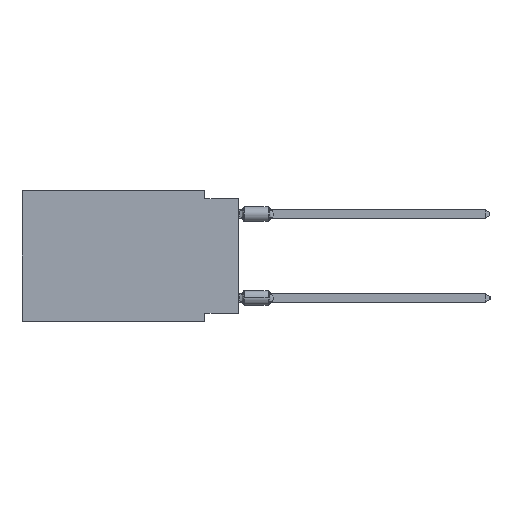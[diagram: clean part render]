
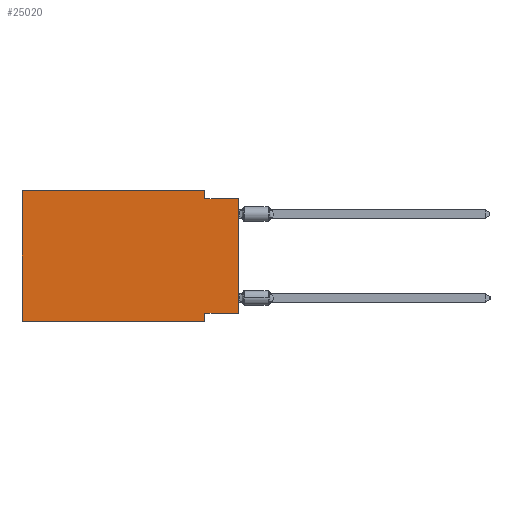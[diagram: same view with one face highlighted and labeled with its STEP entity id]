
A CAD part, left-side view. The second image highlights one B-rep face of the part: STEP entity #25020.
In plain terms, the highlighted planar face has unit normal (-1, 0, 0).
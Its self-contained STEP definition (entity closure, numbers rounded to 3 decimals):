
#101 = EDGE_CURVE ( 'NONE', #22344, #44225, #12559, .T. ) ;
#340 = AXIS2_PLACEMENT_3D ( 'NONE', #10035, #46020, #37807 ) ;
#883 = DIRECTION ( 'NONE',  ( 0., 0., 1. ) ) ;
#992 = EDGE_CURVE ( 'NONE', #17172, #22344, #31655, .T. ) ;
#3326 = CARTESIAN_POINT ( 'NONE',  ( 0., 2.54, -0.635 ) ) ;
#3798 = VERTEX_POINT ( 'NONE', #25365 ) ;
#3814 = VECTOR ( 'NONE', #20642, 1000. ) ;
#4073 = ORIENTED_EDGE ( 'NONE', *, *, #49461, .T. ) ;
#4713 = CARTESIAN_POINT ( 'NONE',  ( 0., 2.54, -9.271 ) ) ;
#7022 = ORIENTED_EDGE ( 'NONE', *, *, #101, .F. ) ;
#10035 = CARTESIAN_POINT ( 'NONE',  ( 0., 16.383, 0. ) ) ;
#10732 = DIRECTION ( 'NONE',  ( 0., 0., -1. ) ) ;
#11521 = ORIENTED_EDGE ( 'NONE', *, *, #28803, .F. ) ;
#11645 = EDGE_LOOP ( 'NONE', ( #25364, #38021, #7022, #18798, #50456, #4073, #11521, #11876 ) ) ;
#11876 = ORIENTED_EDGE ( 'NONE', *, *, #16154, .F. ) ;
#12080 = VECTOR ( 'NONE', #883, 1000. ) ;
#12559 = LINE ( 'NONE', #19753, #28662 ) ;
#12945 = LINE ( 'NONE', #28630, #12080 ) ;
#13032 = VECTOR ( 'NONE', #44500, 1000. ) ;
#13694 = CARTESIAN_POINT ( 'NONE',  ( 0., 16.383, -9.906 ) ) ;
#14316 = LINE ( 'NONE', #34862, #21772 ) ;
#16154 = EDGE_CURVE ( 'NONE', #3798, #38012, #21662, .T. ) ;
#16664 = DIRECTION ( 'NONE',  ( 0., 0., -1. ) ) ;
#17172 = VERTEX_POINT ( 'NONE', #18712 ) ;
#17536 = CARTESIAN_POINT ( 'NONE',  ( 0., 16.383, -9.906 ) ) ;
#18712 = CARTESIAN_POINT ( 'NONE',  ( 0., 16.383, 0. ) ) ;
#18798 = ORIENTED_EDGE ( 'NONE', *, *, #992, .F. ) ;
#19212 = CARTESIAN_POINT ( 'NONE',  ( 0., 2.54, 0. ) ) ;
#19753 = CARTESIAN_POINT ( 'NONE',  ( 0., 2.54, 0. ) ) ;
#20642 = DIRECTION ( 'NONE',  ( 0., 0., 1. ) ) ;
#21662 = LINE ( 'NONE', #32544, #37453 ) ;
#21772 = VECTOR ( 'NONE', #10732, 1000. ) ;
#22344 = VERTEX_POINT ( 'NONE', #19212 ) ;
#23284 = EDGE_CURVE ( 'NONE', #44225, #39019, #31977, .T. ) ;
#24594 = DIRECTION ( 'NONE',  ( 0., 1., 0. ) ) ;
#24997 = LINE ( 'NONE', #17536, #34385 ) ;
#25020 = ADVANCED_FACE ( 'NONE', ( #33933 ), #30350, .F. ) ;
#25364 = ORIENTED_EDGE ( 'NONE', *, *, #35558, .T. ) ;
#25365 = CARTESIAN_POINT ( 'NONE',  ( 0., 0., -9.271 ) ) ;
#26861 = CARTESIAN_POINT ( 'NONE',  ( 0., 0., -0.635 ) ) ;
#27562 = LINE ( 'NONE', #35307, #3814 ) ;
#28630 = CARTESIAN_POINT ( 'NONE',  ( 0., 16.383, 0. ) ) ;
#28662 = VECTOR ( 'NONE', #16664, 1000. ) ;
#28803 = EDGE_CURVE ( 'NONE', #38012, #34440, #14316, .T. ) ;
#29475 = VERTEX_POINT ( 'NONE', #13694 ) ;
#29481 = VECTOR ( 'NONE', #47650, 1000. ) ;
#30350 = PLANE ( 'NONE',  #340 ) ;
#31655 = LINE ( 'NONE', #47333, #13032 ) ;
#31977 = LINE ( 'NONE', #43772, #29481 ) ;
#32544 = CARTESIAN_POINT ( 'NONE',  ( 0., 0., -9.271 ) ) ;
#33109 = EDGE_CURVE ( 'NONE', #29475, #17172, #12945, .T. ) ;
#33933 = FACE_OUTER_BOUND ( 'NONE', #11645, .T. ) ;
#34385 = VECTOR ( 'NONE', #36584, 1000. ) ;
#34440 = VERTEX_POINT ( 'NONE', #44553 ) ;
#34862 = CARTESIAN_POINT ( 'NONE',  ( 0., 2.54, -9.906 ) ) ;
#35307 = CARTESIAN_POINT ( 'NONE',  ( 0., 0., 0. ) ) ;
#35558 = EDGE_CURVE ( 'NONE', #3798, #39019, #27562, .T. ) ;
#36584 = DIRECTION ( 'NONE',  ( 0., -1., 0. ) ) ;
#37453 = VECTOR ( 'NONE', #24594, 1000. ) ;
#37807 = DIRECTION ( 'NONE',  ( 0., 0., -1. ) ) ;
#38012 = VERTEX_POINT ( 'NONE', #4713 ) ;
#38021 = ORIENTED_EDGE ( 'NONE', *, *, #23284, .F. ) ;
#39019 = VERTEX_POINT ( 'NONE', #26861 ) ;
#43772 = CARTESIAN_POINT ( 'NONE',  ( 0., 0., -0.635 ) ) ;
#44225 = VERTEX_POINT ( 'NONE', #3326 ) ;
#44500 = DIRECTION ( 'NONE',  ( 0., -1., 0. ) ) ;
#44553 = CARTESIAN_POINT ( 'NONE',  ( 0., 2.54, -9.906 ) ) ;
#46020 = DIRECTION ( 'NONE',  ( 1., 0., 0. ) ) ;
#47333 = CARTESIAN_POINT ( 'NONE',  ( 0., 16.383, 0. ) ) ;
#47650 = DIRECTION ( 'NONE',  ( 0., -1., 0. ) ) ;
#49461 = EDGE_CURVE ( 'NONE', #29475, #34440, #24997, .T. ) ;
#50456 = ORIENTED_EDGE ( 'NONE', *, *, #33109, .F. ) ;
